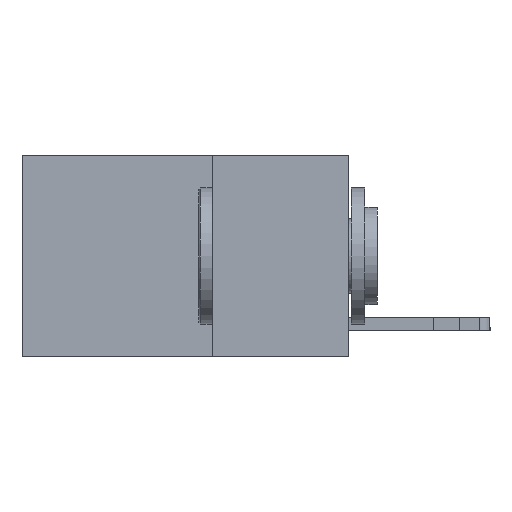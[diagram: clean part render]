
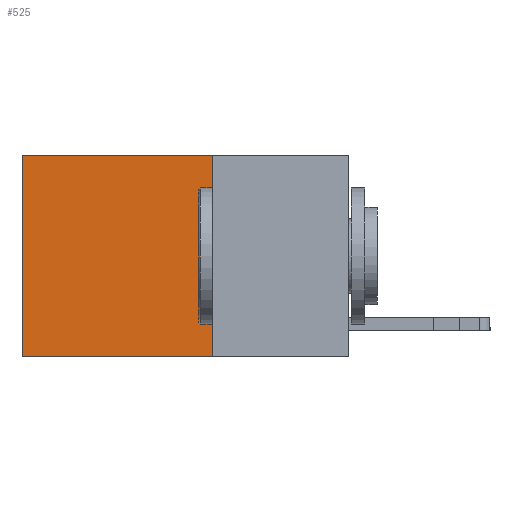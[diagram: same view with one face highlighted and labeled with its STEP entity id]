
A CAD part, left-side view. The second image highlights one B-rep face of the part: STEP entity #525.
In plain terms, the highlighted planar face has unit normal (-1, 0, 0).
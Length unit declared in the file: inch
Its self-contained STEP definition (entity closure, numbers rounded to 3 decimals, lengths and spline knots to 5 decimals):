
#525 = ADVANCED_FACE ( 'NONE', ( #12420 ), #12277, .F. ) ;
#1053 = VECTOR ( 'NONE', #12103, 39.37008 ) ;
#1291 = CARTESIAN_POINT ( 'NONE',  ( 0.2625, 0.6, 0. ) ) ;
#1869 = CARTESIAN_POINT ( 'NONE',  ( 0.2625, 0.25, 0. ) ) ;
#1942 = DIRECTION ( 'NONE',  ( 0., 0., -1. ) ) ;
#2221 = DIRECTION ( 'NONE',  ( 0., 0., -1. ) ) ;
#2299 = LINE ( 'NONE', #7662, #12424 ) ;
#2472 = CARTESIAN_POINT ( 'NONE',  ( 0.2625, 0.25, 0. ) ) ;
#3554 = EDGE_LOOP ( 'NONE', ( #11156, #10389, #5689, #10238 ) ) ;
#4159 = CARTESIAN_POINT ( 'NONE',  ( 0.2625, 0.25, 0. ) ) ;
#5048 = CARTESIAN_POINT ( 'NONE',  ( 0.2625, 0.25, -0.37 ) ) ;
#5119 = CARTESIAN_POINT ( 'NONE',  ( 0.2625, 0.6, -0.37 ) ) ;
#5183 = DIRECTION ( 'NONE',  ( 0., 0., -1. ) ) ;
#5184 = LINE ( 'NONE', #4159, #11848 ) ;
#5689 = ORIENTED_EDGE ( 'NONE', *, *, #13147, .F. ) ;
#6509 = CARTESIAN_POINT ( 'NONE',  ( 0.2625, 0.25, -0.37 ) ) ;
#6793 = VERTEX_POINT ( 'NONE', #2472 ) ;
#7169 = DIRECTION ( 'NONE',  ( 1., 0., 0. ) ) ;
#7662 = CARTESIAN_POINT ( 'NONE',  ( 0.2625, 0.6, 0. ) ) ;
#7796 = LINE ( 'NONE', #6509, #12726 ) ;
#7894 = EDGE_CURVE ( 'NONE', #6793, #9920, #10003, .T. ) ;
#8057 = EDGE_CURVE ( 'NONE', #9920, #12036, #2299, .T. ) ;
#8613 = DIRECTION ( 'NONE',  ( 0., 1., 0. ) ) ;
#9857 = CARTESIAN_POINT ( 'NONE',  ( 0.2625, 0.25, 0. ) ) ;
#9920 = VERTEX_POINT ( 'NONE', #1291 ) ;
#10003 = LINE ( 'NONE', #9857, #1053 ) ;
#10238 = ORIENTED_EDGE ( 'NONE', *, *, #7894, .T. ) ;
#10389 = ORIENTED_EDGE ( 'NONE', *, *, #12902, .F. ) ;
#11156 = ORIENTED_EDGE ( 'NONE', *, *, #8057, .T. ) ;
#11848 = VECTOR ( 'NONE', #1942, 39.37008 ) ;
#12036 = VERTEX_POINT ( 'NONE', #5119 ) ;
#12103 = DIRECTION ( 'NONE',  ( 0., 1., 0. ) ) ;
#12277 = PLANE ( 'NONE',  #12324 ) ;
#12324 = AXIS2_PLACEMENT_3D ( 'NONE', #1869, #7169, #5183 ) ;
#12420 = FACE_OUTER_BOUND ( 'NONE', #3554, .T. ) ;
#12424 = VECTOR ( 'NONE', #2221, 39.37008 ) ;
#12726 = VECTOR ( 'NONE', #8613, 39.37008 ) ;
#12902 = EDGE_CURVE ( 'NONE', #13127, #12036, #7796, .T. ) ;
#13127 = VERTEX_POINT ( 'NONE', #5048 ) ;
#13147 = EDGE_CURVE ( 'NONE', #6793, #13127, #5184, .T. ) ;
